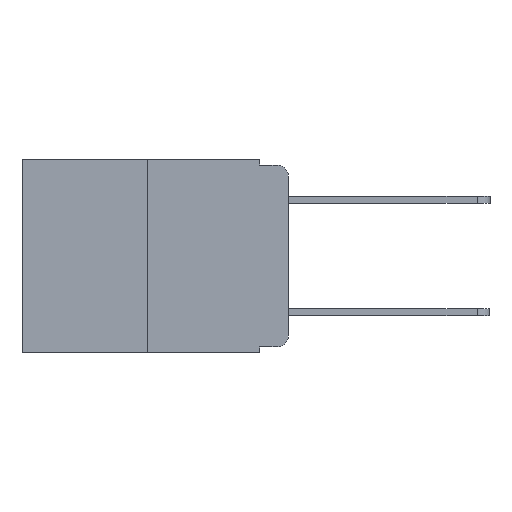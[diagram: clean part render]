
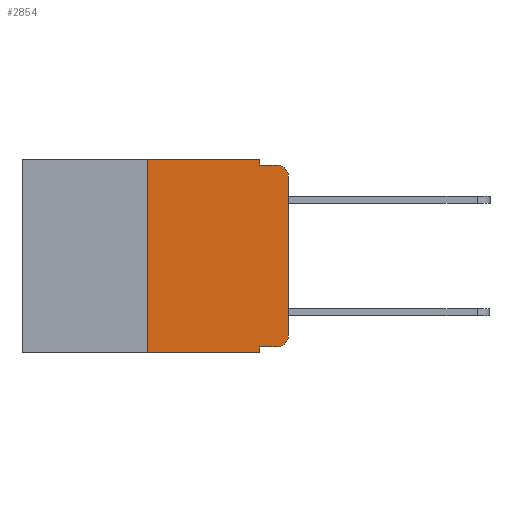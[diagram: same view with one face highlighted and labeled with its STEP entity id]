
A CAD part, left-side view. The second image highlights one B-rep face of the part: STEP entity #2854.
In plain terms, the highlighted planar face has unit normal (-1, 0, 0).
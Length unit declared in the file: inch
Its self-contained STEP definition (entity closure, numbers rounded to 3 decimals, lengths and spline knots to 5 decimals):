
#204 = CARTESIAN_POINT ( 'NONE',  ( 0., 0.473, -0.343 ) ) ;
#499 = CIRCLE ( 'NONE', #7330, 0.02 ) ;
#1017 = VECTOR ( 'NONE', #11922, 39.37008 ) ;
#1219 = LINE ( 'NONE', #10753, #6189 ) ;
#1433 = EDGE_LOOP ( 'NONE', ( #2537, #1455, #10064, #5838, #8037, #5468, #11268, #7973, #7488, #10317 ) ) ;
#1455 = ORIENTED_EDGE ( 'NONE', *, *, #9476, .T. ) ;
#1482 = CIRCLE ( 'NONE', #3322, 0.02 ) ;
#1833 = CARTESIAN_POINT ( 'NONE',  ( 0., 0.02, -0.313 ) ) ;
#1861 = EDGE_CURVE ( 'NONE', #2404, #4693, #6009, .T. ) ;
#1991 = DIRECTION ( 'NONE',  ( 0., -1., 0. ) ) ;
#2019 = EDGE_CURVE ( 'NONE', #8420, #3041, #4495, .T. ) ;
#2122 = DIRECTION ( 'NONE',  ( -1., 0., 0. ) ) ;
#2360 = VECTOR ( 'NONE', #10653, 39.37008 ) ;
#2404 = VERTEX_POINT ( 'NONE', #8432 ) ;
#2507 = CARTESIAN_POINT ( 'NONE',  ( 0., 0.051, 0. ) ) ;
#2537 = ORIENTED_EDGE ( 'NONE', *, *, #1861, .T. ) ;
#2701 = VERTEX_POINT ( 'NONE', #3522 ) ;
#2854 = ADVANCED_FACE ( 'NONE', ( #5485 ), #10919, .F. ) ;
#2889 = DIRECTION ( 'NONE',  ( 0., 0., -1. ) ) ;
#3041 = VERTEX_POINT ( 'NONE', #9061 ) ;
#3322 = AXIS2_PLACEMENT_3D ( 'NONE', #1833, #8502, #2889 ) ;
#3457 = CARTESIAN_POINT ( 'NONE',  ( 0., 0.051, 0. ) ) ;
#3522 = CARTESIAN_POINT ( 'NONE',  ( 0., 0.02, -0.01 ) ) ;
#3709 = LINE ( 'NONE', #5886, #8347 ) ;
#3997 = EDGE_CURVE ( 'NONE', #8239, #7156, #1219, .T. ) ;
#4139 = DIRECTION ( 'NONE',  ( 0., 0., -1. ) ) ;
#4152 = EDGE_CURVE ( 'NONE', #5010, #2701, #9256, .T. ) ;
#4495 = LINE ( 'NONE', #5744, #6693 ) ;
#4502 = CARTESIAN_POINT ( 'NONE',  ( 0., 0.051, -0.01 ) ) ;
#4693 = VERTEX_POINT ( 'NONE', #5423 ) ;
#4847 = CARTESIAN_POINT ( 'NONE',  ( 0., 0.051, 0. ) ) ;
#5010 = VERTEX_POINT ( 'NONE', #9943 ) ;
#5141 = VERTEX_POINT ( 'NONE', #4847 ) ;
#5423 = CARTESIAN_POINT ( 'NONE',  ( 0., 0., -0.03 ) ) ;
#5468 = ORIENTED_EDGE ( 'NONE', *, *, #3997, .F. ) ;
#5485 = FACE_OUTER_BOUND ( 'NONE', #1433, .T. ) ;
#5744 = CARTESIAN_POINT ( 'NONE',  ( 0., 0.051, -0.333 ) ) ;
#5838 = ORIENTED_EDGE ( 'NONE', *, *, #11500, .F. ) ;
#5886 = CARTESIAN_POINT ( 'NONE',  ( 0., 0.473, 0. ) ) ;
#6009 = LINE ( 'NONE', #9826, #1017 ) ;
#6189 = VECTOR ( 'NONE', #11146, 39.37008 ) ;
#6693 = VECTOR ( 'NONE', #10880, 39.37008 ) ;
#6717 = VERTEX_POINT ( 'NONE', #9459 ) ;
#7156 = VERTEX_POINT ( 'NONE', #8224 ) ;
#7330 = AXIS2_PLACEMENT_3D ( 'NONE', #7818, #2122, #8719 ) ;
#7426 = LINE ( 'NONE', #2507, #2360 ) ;
#7488 = ORIENTED_EDGE ( 'NONE', *, *, #2019, .T. ) ;
#7525 = EDGE_CURVE ( 'NONE', #7156, #5141, #3709, .T. ) ;
#7818 = CARTESIAN_POINT ( 'NONE',  ( 0., 0.02, -0.03 ) ) ;
#7973 = ORIENTED_EDGE ( 'NONE', *, *, #8311, .F. ) ;
#8037 = ORIENTED_EDGE ( 'NONE', *, *, #7525, .F. ) ;
#8224 = CARTESIAN_POINT ( 'NONE',  ( 0., 0.25, 0. ) ) ;
#8239 = VERTEX_POINT ( 'NONE', #8937 ) ;
#8311 = EDGE_CURVE ( 'NONE', #8420, #6717, #7426, .T. ) ;
#8347 = VECTOR ( 'NONE', #1991, 39.37008 ) ;
#8355 = DIRECTION ( 'NONE',  ( 0., -1., 0. ) ) ;
#8420 = VERTEX_POINT ( 'NONE', #11645 ) ;
#8432 = CARTESIAN_POINT ( 'NONE',  ( 0., 0., -0.313 ) ) ;
#8502 = DIRECTION ( 'NONE',  ( -1., 0., 0. ) ) ;
#8719 = DIRECTION ( 'NONE',  ( 0., 0., -1. ) ) ;
#8937 = CARTESIAN_POINT ( 'NONE',  ( 0., 0.25, -0.343 ) ) ;
#8960 = EDGE_CURVE ( 'NONE', #8239, #6717, #10512, .T. ) ;
#8982 = VECTOR ( 'NONE', #8355, 39.37008 ) ;
#8983 = DIRECTION ( 'NONE',  ( 0., 0., -1. ) ) ;
#9061 = CARTESIAN_POINT ( 'NONE',  ( 0., 0.02, -0.333 ) ) ;
#9256 = LINE ( 'NONE', #4502, #8982 ) ;
#9459 = CARTESIAN_POINT ( 'NONE',  ( 0., 0.051, -0.343 ) ) ;
#9476 = EDGE_CURVE ( 'NONE', #4693, #2701, #499, .T. ) ;
#9573 = LINE ( 'NONE', #3457, #11753 ) ;
#9809 = DIRECTION ( 'NONE',  ( 0., -1., 0. ) ) ;
#9826 = CARTESIAN_POINT ( 'NONE',  ( 0., 0., 0. ) ) ;
#9894 = EDGE_CURVE ( 'NONE', #3041, #2404, #1482, .T. ) ;
#9943 = CARTESIAN_POINT ( 'NONE',  ( 0., 0.051, -0.01 ) ) ;
#10064 = ORIENTED_EDGE ( 'NONE', *, *, #4152, .F. ) ;
#10259 = VECTOR ( 'NONE', #9809, 39.37008 ) ;
#10317 = ORIENTED_EDGE ( 'NONE', *, *, #9894, .T. ) ;
#10512 = LINE ( 'NONE', #204, #10259 ) ;
#10653 = DIRECTION ( 'NONE',  ( 0., 0., -1. ) ) ;
#10753 = CARTESIAN_POINT ( 'NONE',  ( 0., 0.25, 0. ) ) ;
#10851 = DIRECTION ( 'NONE',  ( 1., 0., 0. ) ) ;
#10880 = DIRECTION ( 'NONE',  ( 0., -1., 0. ) ) ;
#10919 = PLANE ( 'NONE',  #11935 ) ;
#11146 = DIRECTION ( 'NONE',  ( 0., 0., 1. ) ) ;
#11268 = ORIENTED_EDGE ( 'NONE', *, *, #8960, .T. ) ;
#11279 = CARTESIAN_POINT ( 'NONE',  ( 0., 0.473, 0. ) ) ;
#11500 = EDGE_CURVE ( 'NONE', #5141, #5010, #9573, .T. ) ;
#11645 = CARTESIAN_POINT ( 'NONE',  ( 0., 0.051, -0.333 ) ) ;
#11753 = VECTOR ( 'NONE', #8983, 39.37008 ) ;
#11922 = DIRECTION ( 'NONE',  ( 0., 0., 1. ) ) ;
#11935 = AXIS2_PLACEMENT_3D ( 'NONE', #11279, #10851, #4139 ) ;
